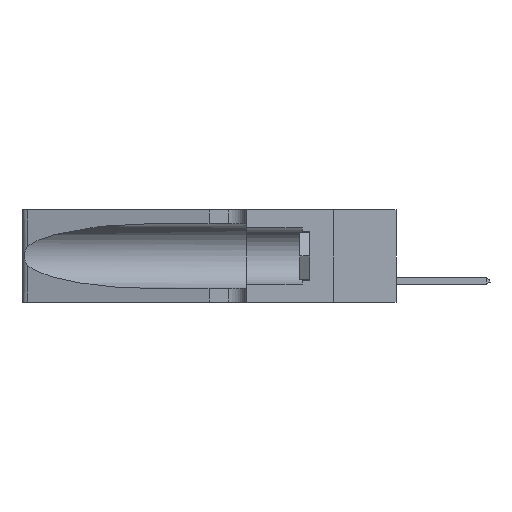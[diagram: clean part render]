
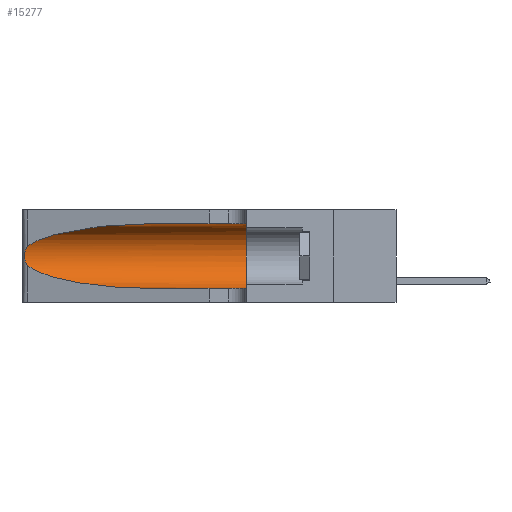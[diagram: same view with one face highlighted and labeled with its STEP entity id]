
A CAD part, left-side view. The second image highlights one B-rep face of the part: STEP entity #15277.
In plain terms, the highlighted cylindrical face has radius 3.308 mm (diameter 6.617 mm), a partial arc.
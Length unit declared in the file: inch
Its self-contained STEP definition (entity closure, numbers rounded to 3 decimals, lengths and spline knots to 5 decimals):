
#1463 = ORIENTED_EDGE ( 'NONE', *, *, #18089, .T. ) ;
#3249 = CARTESIAN_POINT ( 'NONE',  ( 0.1305, 0.72297, 0.31525 ) ) ;
#3441 = EDGE_CURVE ( 'NONE', #42629, #18734, #47224, .T. ) ;
#3636 = VERTEX_POINT ( 'NONE', #5786 ) ;
#4666 = CARTESIAN_POINT ( 'NONE',  ( 0.25555, 1.22993, 0.14849 ) ) ;
#5493 = FACE_OUTER_BOUND ( 'NONE', #26148, .T. ) ;
#5786 = CARTESIAN_POINT ( 'NONE',  ( 0.1305, 0.35, 0.05475 ) ) ;
#7817 = CARTESIAN_POINT ( 'NONE',  ( 0.1305, 0.35, 0.31525 ) ) ;
#7873 = CARTESIAN_POINT ( 'NONE',  ( 0.25854, 1.2359, 0.20912 ) ) ;
#8052 = CARTESIAN_POINT ( 'NONE',  ( 0.25555, 1.22994, 0.2215 ) ) ;
#8204 = CARTESIAN_POINT ( 'NONE',  ( 0.25856, 1.23593, 0.16098 ) ) ;
#9934 = CARTESIAN_POINT ( 'NONE',  ( 0.25487, 1.22718, 0.14631 ) ) ;
#10092 = CARTESIAN_POINT ( 'NONE',  ( 0.18966, 0.96281, 0.05475 ) ) ;
#10630 = CARTESIAN_POINT ( 'NONE',  ( 0.1305, 1.61858, 0.185 ) ) ;
#11291 = CYLINDRICAL_SURFACE ( 'NONE', #43447, 0.13025 ) ;
#11298 = CARTESIAN_POINT ( 'NONE',  ( 0.26017, 1.23833, 0.17102 ) ) ;
#11524 = VECTOR ( 'NONE', #42199, 39.37008 ) ;
#11892 = LINE ( 'NONE', #31068, #16540 ) ;
#12347 = CARTESIAN_POINT ( 'NONE',  ( 0.1305, 1.61858, 0.05475 ) ) ;
#12561 = CARTESIAN_POINT ( 'NONE',  ( 0.25487, 1.22718, 0.14631 ) ) ;
#15277 = ADVANCED_FACE ( 'NONE', ( #5493 ), #11291, .F. ) ;
#16540 = VECTOR ( 'NONE', #35647, 39.37008 ) ;
#17533 = CARTESIAN_POINT ( 'NONE',  ( 0.1305, 0.72297, 0.05475 ) ) ;
#17952 = EDGE_CURVE ( 'NONE', #44401, #42629, #41338, .T. ) ;
#18089 = EDGE_CURVE ( 'NONE', #18734, #26588, #21366, .T. ) ;
#18249 = EDGE_CURVE ( 'NONE', #26588, #3636, #31773, .T. ) ;
#18572 = EDGE_CURVE ( 'NONE', #38892, #3636, #25373, .T. ) ;
#18734 = VERTEX_POINT ( 'NONE', #25588 ) ;
#19611 = DIRECTION ( 'NONE',  ( 0., -1., 0. ) ) ;
#19776 = DIRECTION ( 'NONE',  ( 0., 0., -1. ) ) ;
#21366 =( BOUNDED_CURVE ( )  B_SPLINE_CURVE ( 3, ( #9934, #43325, #10092, #17533 ),
 .UNSPECIFIED., .F., .F. ) 
 B_SPLINE_CURVE_WITH_KNOTS ( ( 4, 4 ),
 ( 3.44316, 4.71239 ),
 .UNSPECIFIED. ) 
 CURVE ( )  GEOMETRIC_REPRESENTATION_ITEM ( )  RATIONAL_B_SPLINE_CURVE ( ( 1., 0.87, 0.87, 1. ) ) 
 REPRESENTATION_ITEM ( '' )  );
#22035 = DIRECTION ( 'NONE',  ( 0., 1., 0. ) ) ;
#22922 = CARTESIAN_POINT ( 'NONE',  ( 0.26075, 1.23896, 0.19203 ) ) ;
#23665 = CARTESIAN_POINT ( 'NONE',  ( 0.25487, 1.22718, 0.22369 ) ) ;
#25335 = EDGE_CURVE ( 'NONE', #44401, #38892, #11892, .T. ) ;
#25373 = CIRCLE ( 'NONE', #47240, 0.13025 ) ;
#25588 = CARTESIAN_POINT ( 'NONE',  ( 0.25487, 1.22718, 0.14631 ) ) ;
#26148 = EDGE_LOOP ( 'NONE', ( #34099, #36016, #1463, #28059, #32162, #31810 ) ) ;
#26588 = VERTEX_POINT ( 'NONE', #34804 ) ;
#28059 = ORIENTED_EDGE ( 'NONE', *, *, #18249, .T. ) ;
#30247 = CARTESIAN_POINT ( 'NONE',  ( 0.25487, 1.22718, 0.22369 ) ) ;
#30393 = CARTESIAN_POINT ( 'NONE',  ( 0.26075, 1.23896, 0.178 ) ) ;
#31068 = CARTESIAN_POINT ( 'NONE',  ( 0.1305, 1.61858, 0.31525 ) ) ;
#31773 = LINE ( 'NONE', #12347, #11524 ) ;
#31810 = ORIENTED_EDGE ( 'NONE', *, *, #25335, .F. ) ;
#32162 = ORIENTED_EDGE ( 'NONE', *, *, #18572, .F. ) ;
#33044 = CARTESIAN_POINT ( 'NONE',  ( 0.1305, 0.35, 0.185 ) ) ;
#33620 = CARTESIAN_POINT ( 'NONE',  ( 0.25787, 1.23484, 0.2124 ) ) ;
#34099 = ORIENTED_EDGE ( 'NONE', *, *, #17952, .T. ) ;
#34437 = CARTESIAN_POINT ( 'NONE',  ( 0.25639, 1.23186, 0.15144 ) ) ;
#34619 = CARTESIAN_POINT ( 'NONE',  ( 0.25487, 1.22718, 0.22369 ) ) ;
#34804 = CARTESIAN_POINT ( 'NONE',  ( 0.1305, 0.72297, 0.05475 ) ) ;
#35647 = DIRECTION ( 'NONE',  ( 0., -1., 0. ) ) ;
#36016 = ORIENTED_EDGE ( 'NONE', *, *, #3441, .T. ) ;
#38365 = CARTESIAN_POINT ( 'NONE',  ( 0.25789, 1.23486, 0.15765 ) ) ;
#38472 = CARTESIAN_POINT ( 'NONE',  ( 0.18966, 0.96281, 0.31525 ) ) ;
#38892 = VERTEX_POINT ( 'NONE', #7817 ) ;
#40877 = DIRECTION ( 'NONE',  ( 0., 0., 1. ) ) ;
#41248 = CARTESIAN_POINT ( 'NONE',  ( 0.1305, 0.72297, 0.31525 ) ) ;
#41338 =( BOUNDED_CURVE ( )  B_SPLINE_CURVE ( 3, ( #41248, #38472, #42198, #23665 ),
 .UNSPECIFIED., .F., .F. ) 
 B_SPLINE_CURVE_WITH_KNOTS ( ( 4, 4 ),
 ( 1.5708, 2.84003 ),
 .UNSPECIFIED. ) 
 CURVE ( )  GEOMETRIC_REPRESENTATION_ITEM ( )  RATIONAL_B_SPLINE_CURVE ( ( 1., 0.87, 0.87, 1. ) ) 
 REPRESENTATION_ITEM ( '' )  );
#41453 = CARTESIAN_POINT ( 'NONE',  ( 0.25639, 1.23184, 0.21858 ) ) ;
#42198 = CARTESIAN_POINT ( 'NONE',  ( 0.2373, 1.15595, 0.28018 ) ) ;
#42199 = DIRECTION ( 'NONE',  ( 0., -1., 0. ) ) ;
#42629 = VERTEX_POINT ( 'NONE', #34619 ) ;
#43325 = CARTESIAN_POINT ( 'NONE',  ( 0.2373, 1.15595, 0.08982 ) ) ;
#43447 = AXIS2_PLACEMENT_3D ( 'NONE', #10630, #19611, #19776 ) ;
#44401 = VERTEX_POINT ( 'NONE', #3249 ) ;
#45122 = CARTESIAN_POINT ( 'NONE',  ( 0.26018, 1.23835, 0.19895 ) ) ;
#47224 = B_SPLINE_CURVE_WITH_KNOTS ( 'NONE', 3,
 ( #30247, #8052, #41453, #33620, #7873, #45122, #22922, #30393, #11298, #8204, #38365, #34437, #4666, #12561 ),
 .UNSPECIFIED., .F., .F.,
 ( 4, 2, 2, 2, 2, 2, 4 ),
 ( 0., 0.00027, 0.00053, 0.00107, 0.0016, 0.00187, 0.00214 ),
 .UNSPECIFIED. ) ;
#47240 = AXIS2_PLACEMENT_3D ( 'NONE', #33044, #22035, #40877 ) ;
